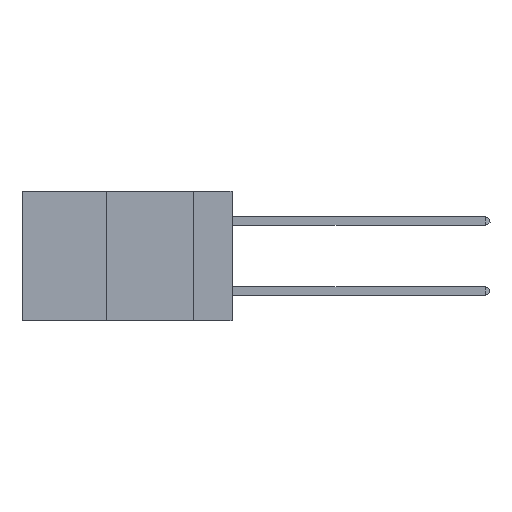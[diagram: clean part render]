
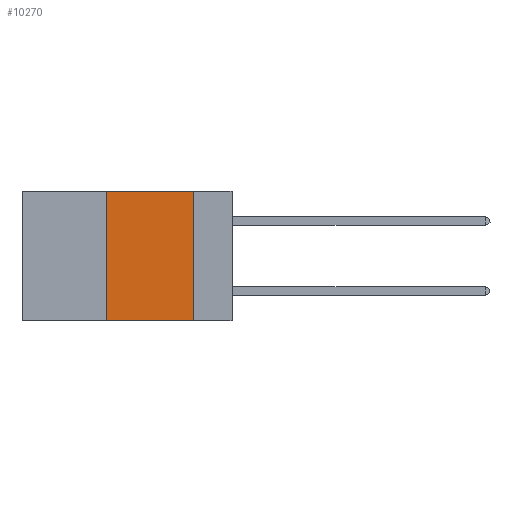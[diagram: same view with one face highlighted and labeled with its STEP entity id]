
A CAD part, left-side view. The second image highlights one B-rep face of the part: STEP entity #10270.
In plain terms, the highlighted planar face has unit normal (-1, 0, 0).
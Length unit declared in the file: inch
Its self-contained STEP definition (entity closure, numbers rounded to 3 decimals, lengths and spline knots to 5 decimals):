
#763 = VECTOR ( 'NONE', #10472, 39.37008 ) ;
#872 = ORIENTED_EDGE ( 'NONE', *, *, #2839, .F. ) ;
#1012 = EDGE_CURVE ( 'NONE', #7841, #13247, #6329, .T. ) ;
#1165 = DIRECTION ( 'NONE',  ( 0., -1., 0. ) ) ;
#2645 = CARTESIAN_POINT ( 'NONE',  ( 0., 0.11, 0. ) ) ;
#2671 = LINE ( 'NONE', #4777, #763 ) ;
#2820 = ORIENTED_EDGE ( 'NONE', *, *, #1012, .T. ) ;
#2839 = EDGE_CURVE ( 'NONE', #3048, #13247, #12217, .T. ) ;
#2912 = DIRECTION ( 'NONE',  ( 1., 0., 0. ) ) ;
#3048 = VERTEX_POINT ( 'NONE', #9631 ) ;
#3050 = VECTOR ( 'NONE', #4610, 39.37008 ) ;
#3512 = CARTESIAN_POINT ( 'NONE',  ( 0., 0.36, 0. ) ) ;
#3794 = EDGE_LOOP ( 'NONE', ( #872, #4284, #10029, #2820 ) ) ;
#3933 = DIRECTION ( 'NONE',  ( 0., 0., -1. ) ) ;
#4284 = ORIENTED_EDGE ( 'NONE', *, *, #10877, .F. ) ;
#4487 = AXIS2_PLACEMENT_3D ( 'NONE', #8231, #2912, #13485 ) ;
#4610 = DIRECTION ( 'NONE',  ( 0., 0., 1. ) ) ;
#4777 = CARTESIAN_POINT ( 'NONE',  ( 0., 0.6, 0. ) ) ;
#5624 = VECTOR ( 'NONE', #3933, 39.37008 ) ;
#6168 = VECTOR ( 'NONE', #1165, 39.37008 ) ;
#6329 = LINE ( 'NONE', #9755, #6168 ) ;
#7194 = CARTESIAN_POINT ( 'NONE',  ( 0., 0.36, 0. ) ) ;
#7841 = VERTEX_POINT ( 'NONE', #10611 ) ;
#8043 = VERTEX_POINT ( 'NONE', #7194 ) ;
#8231 = CARTESIAN_POINT ( 'NONE',  ( 0., 0.6, 0. ) ) ;
#9631 = CARTESIAN_POINT ( 'NONE',  ( 0., 0.11, 0. ) ) ;
#9755 = CARTESIAN_POINT ( 'NONE',  ( 0., 0.6, -0.37 ) ) ;
#10029 = ORIENTED_EDGE ( 'NONE', *, *, #13662, .F. ) ;
#10139 = LINE ( 'NONE', #3512, #3050 ) ;
#10270 = ADVANCED_FACE ( 'NONE', ( #11429 ), #13444, .F. ) ;
#10472 = DIRECTION ( 'NONE',  ( 0., -1., 0. ) ) ;
#10611 = CARTESIAN_POINT ( 'NONE',  ( 0., 0.36, -0.37 ) ) ;
#10877 = EDGE_CURVE ( 'NONE', #8043, #3048, #2671, .T. ) ;
#11408 = CARTESIAN_POINT ( 'NONE',  ( 0., 0.11, -0.37 ) ) ;
#11429 = FACE_OUTER_BOUND ( 'NONE', #3794, .T. ) ;
#12217 = LINE ( 'NONE', #2645, #5624 ) ;
#13247 = VERTEX_POINT ( 'NONE', #11408 ) ;
#13444 = PLANE ( 'NONE',  #4487 ) ;
#13485 = DIRECTION ( 'NONE',  ( 0., 0., -1. ) ) ;
#13662 = EDGE_CURVE ( 'NONE', #7841, #8043, #10139, .T. ) ;
